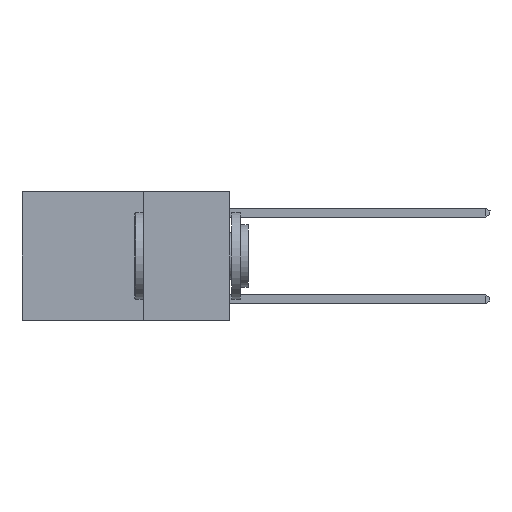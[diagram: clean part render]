
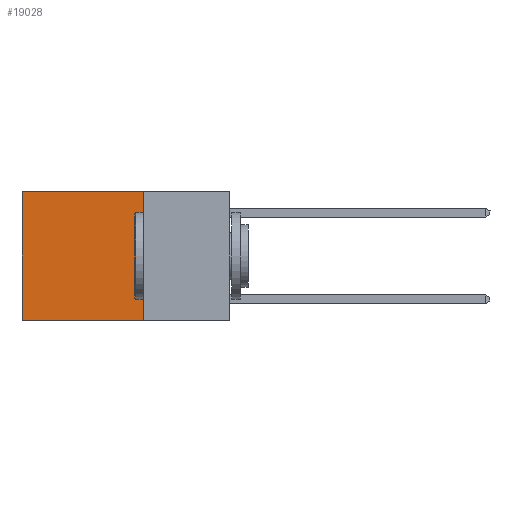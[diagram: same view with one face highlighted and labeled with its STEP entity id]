
A CAD part, left-side view. The second image highlights one B-rep face of the part: STEP entity #19028.
In plain terms, the highlighted planar face has unit normal (-1, 0, 0).
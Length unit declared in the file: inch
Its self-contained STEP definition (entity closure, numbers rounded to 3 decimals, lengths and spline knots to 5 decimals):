
#85 = PLANE ( 'NONE',  #12553 ) ;
#351 = FACE_OUTER_BOUND ( 'NONE', #4804, .T. ) ;
#409 = CARTESIAN_POINT ( 'NONE',  ( 0.2625, 0.25, -0.37 ) ) ;
#774 = VERTEX_POINT ( 'NONE', #21801 ) ;
#942 = CARTESIAN_POINT ( 'NONE',  ( 0.2625, 0.6, 0. ) ) ;
#961 = LINE ( 'NONE', #8163, #5504 ) ;
#1976 = DIRECTION ( 'NONE',  ( 1., 0., 0. ) ) ;
#2369 = ORIENTED_EDGE ( 'NONE', *, *, #24889, .T. ) ;
#2468 = LINE ( 'NONE', #409, #5445 ) ;
#2492 = ORIENTED_EDGE ( 'NONE', *, *, #19022, .T. ) ;
#3187 = EDGE_CURVE ( 'NONE', #16628, #774, #2468, .T. ) ;
#4804 = EDGE_LOOP ( 'NONE', ( #2369, #24983, #17323, #2492 ) ) ;
#5445 = VECTOR ( 'NONE', #17803, 39.37008 ) ;
#5504 = VECTOR ( 'NONE', #6103, 39.37008 ) ;
#6103 = DIRECTION ( 'NONE',  ( 0., 1., 0. ) ) ;
#6422 = LINE ( 'NONE', #942, #7950 ) ;
#6706 = VECTOR ( 'NONE', #12525, 39.37008 ) ;
#7950 = VECTOR ( 'NONE', #10423, 39.37008 ) ;
#8163 = CARTESIAN_POINT ( 'NONE',  ( 0.2625, 0.25, 0. ) ) ;
#9707 = LINE ( 'NONE', #24433, #6706 ) ;
#10423 = DIRECTION ( 'NONE',  ( 0., 0., -1. ) ) ;
#10680 = CARTESIAN_POINT ( 'NONE',  ( 0.2625, 0.25, -0.37 ) ) ;
#11889 = DIRECTION ( 'NONE',  ( 0., 0., -1. ) ) ;
#12525 = DIRECTION ( 'NONE',  ( 0., 0., -1. ) ) ;
#12553 = AXIS2_PLACEMENT_3D ( 'NONE', #13759, #1976, #11889 ) ;
#12578 = EDGE_CURVE ( 'NONE', #19348, #16628, #9707, .T. ) ;
#13759 = CARTESIAN_POINT ( 'NONE',  ( 0.2625, 0.25, 0. ) ) ;
#14545 = CARTESIAN_POINT ( 'NONE',  ( 0.2625, 0.6, 0. ) ) ;
#16626 = VERTEX_POINT ( 'NONE', #14545 ) ;
#16628 = VERTEX_POINT ( 'NONE', #10680 ) ;
#17323 = ORIENTED_EDGE ( 'NONE', *, *, #12578, .F. ) ;
#17803 = DIRECTION ( 'NONE',  ( 0., 1., 0. ) ) ;
#19022 = EDGE_CURVE ( 'NONE', #19348, #16626, #961, .T. ) ;
#19028 = ADVANCED_FACE ( 'NONE', ( #351 ), #85, .F. ) ;
#19348 = VERTEX_POINT ( 'NONE', #22112 ) ;
#21801 = CARTESIAN_POINT ( 'NONE',  ( 0.2625, 0.6, -0.37 ) ) ;
#22112 = CARTESIAN_POINT ( 'NONE',  ( 0.2625, 0.25, 0. ) ) ;
#24433 = CARTESIAN_POINT ( 'NONE',  ( 0.2625, 0.25, 0. ) ) ;
#24889 = EDGE_CURVE ( 'NONE', #16626, #774, #6422, .T. ) ;
#24983 = ORIENTED_EDGE ( 'NONE', *, *, #3187, .F. ) ;
